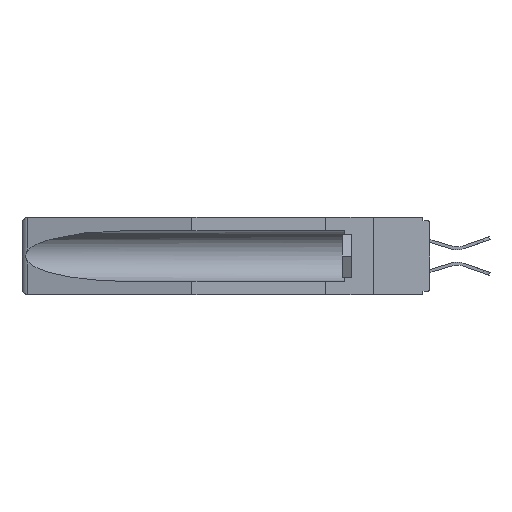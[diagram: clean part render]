
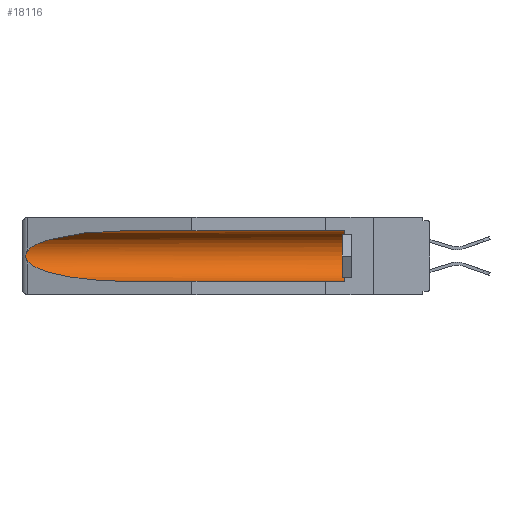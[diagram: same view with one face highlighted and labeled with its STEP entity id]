
A CAD part, left-side view. The second image highlights one B-rep face of the part: STEP entity #18116.
In plain terms, the highlighted cylindrical face has radius 2.857 mm (diameter 5.715 mm), a partial arc.
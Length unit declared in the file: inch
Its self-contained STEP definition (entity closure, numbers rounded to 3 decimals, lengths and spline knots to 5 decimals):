
#35 = CARTESIAN_POINT ( 'NONE',  ( 0.26537, 1.52718, -0.19328 ) ) ;
#506 = CARTESIAN_POINT ( 'NONE',  ( 0.26537, 1.52718, -0.19328 ) ) ;
#765 = CARTESIAN_POINT ( 'NONE',  ( 0.155, 1.07973, -0.059 ) ) ;
#1243 = VERTEX_POINT ( 'NONE', #8244 ) ;
#1831 = VERTEX_POINT ( 'NONE', #11407 ) ;
#2062 = VERTEX_POINT ( 'NONE', #28698 ) ;
#4107 = EDGE_CURVE ( 'NONE', #5020, #1831, #14019, .T. ) ;
#4111 = FACE_OUTER_BOUND ( 'NONE', #20828, .T. ) ;
#4483 = CARTESIAN_POINT ( 'NONE',  ( 0.26537, 1.52718, -0.14972 ) ) ;
#5020 = VERTEX_POINT ( 'NONE', #12432 ) ;
#6721 = CARTESIAN_POINT ( 'NONE',  ( 0.26655, 1.53094, -0.18657 ) ) ;
#6998 = CARTESIAN_POINT ( 'NONE',  ( 0.2675, 1.53308, -0.17534 ) ) ;
#7148 = ORIENTED_EDGE ( 'NONE', *, *, #21753, .T. ) ;
#7287 = CARTESIAN_POINT ( 'NONE',  ( 0.155, -0.30754, -0.284 ) ) ;
#7319 = AXIS2_PLACEMENT_3D ( 'NONE', #10283, #14933, #23999 ) ;
#7691 = VERTEX_POINT ( 'NONE', #10609 ) ;
#8244 = CARTESIAN_POINT ( 'NONE',  ( 0.26537, 1.52718, -0.14972 ) ) ;
#8869 = VERTEX_POINT ( 'NONE', #21587 ) ;
#9433 = EDGE_CURVE ( 'NONE', #1243, #2062, #22752, .T. ) ;
#9462 = EDGE_CURVE ( 'NONE', #2062, #8869, #18335, .T. ) ;
#9974 = CARTESIAN_POINT ( 'NONE',  ( 0.155, -0.30754, -0.059 ) ) ;
#10283 = CARTESIAN_POINT ( 'NONE',  ( 0.155, 0.126, -0.1715 ) ) ;
#10609 = CARTESIAN_POINT ( 'NONE',  ( 0.155, 0.126, -0.284 ) ) ;
#11261 = CARTESIAN_POINT ( 'NONE',  ( 0.26654, 1.53092, -0.15636 ) ) ;
#11364 = CARTESIAN_POINT ( 'NONE',  ( 0.2673, 1.53269, -0.17917 ) ) ;
#11376 = CIRCLE ( 'NONE', #7319, 0.1125 ) ;
#11407 = CARTESIAN_POINT ( 'NONE',  ( 0.155, 1.07973, -0.059 ) ) ;
#11455 = CARTESIAN_POINT ( 'NONE',  ( 0.2673, 1.5327, -0.16383 ) ) ;
#11841 = CARTESIAN_POINT ( 'NONE',  ( 0.155, 1.07973, -0.284 ) ) ;
#12432 = CARTESIAN_POINT ( 'NONE',  ( 0.155, 0.126, -0.059 ) ) ;
#12720 =( BOUNDED_CURVE ( )  B_SPLINE_CURVE ( 3, ( #765, #28111, #14229, #19015 ),
 .UNSPECIFIED., .F., .F. ) 
 B_SPLINE_CURVE_WITH_KNOTS ( ( 4, 4 ),
 ( 4.71239, 6.08839 ),
 .UNSPECIFIED. ) 
 CURVE ( )  GEOMETRIC_REPRESENTATION_ITEM ( )  RATIONAL_B_SPLINE_CURVE ( ( 1., 0.848, 0.848, 1. ) ) 
 REPRESENTATION_ITEM ( '' )  );
#13119 = EDGE_CURVE ( 'NONE', #1831, #1243, #12720, .T. ) ;
#13514 = CARTESIAN_POINT ( 'NONE',  ( 0.2675, 1.53308, -0.16763 ) ) ;
#14019 = LINE ( 'NONE', #9974, #27612 ) ;
#14180 = CARTESIAN_POINT ( 'NONE',  ( 0.21114, 1.30732, -0.284 ) ) ;
#14229 = CARTESIAN_POINT ( 'NONE',  ( 0.25451, 1.48313, -0.09465 ) ) ;
#14885 = DIRECTION ( 'NONE',  ( 0., 0., 1. ) ) ;
#14933 = DIRECTION ( 'NONE',  ( 0., -1., 0. ) ) ;
#15523 = ORIENTED_EDGE ( 'NONE', *, *, #9462, .T. ) ;
#18116 = ADVANCED_FACE ( 'NONE', ( #4111 ), #26829, .F. ) ;
#18335 =( BOUNDED_CURVE ( )  B_SPLINE_CURVE ( 3, ( #506, #22971, #14180, #11841 ),
 .UNSPECIFIED., .F., .F. ) 
 B_SPLINE_CURVE_WITH_KNOTS ( ( 4, 4 ),
 ( 0.1948, 1.5708 ),
 .UNSPECIFIED. ) 
 CURVE ( )  GEOMETRIC_REPRESENTATION_ITEM ( )  RATIONAL_B_SPLINE_CURVE ( ( 1., 0.848, 0.848, 1. ) ) 
 REPRESENTATION_ITEM ( '' )  );
#18692 = DIRECTION ( 'NONE',  ( 0., 1., 0. ) ) ;
#19015 = CARTESIAN_POINT ( 'NONE',  ( 0.26537, 1.52718, -0.14972 ) ) ;
#19338 = CARTESIAN_POINT ( 'NONE',  ( 0.155, -0.30754, -0.1715 ) ) ;
#20357 = ORIENTED_EDGE ( 'NONE', *, *, #9433, .T. ) ;
#20828 = EDGE_LOOP ( 'NONE', ( #27815, #20357, #15523, #23781, #7148, #21472 ) ) ;
#21472 = ORIENTED_EDGE ( 'NONE', *, *, #4107, .T. ) ;
#21587 = CARTESIAN_POINT ( 'NONE',  ( 0.155, 1.07973, -0.284 ) ) ;
#21753 = EDGE_CURVE ( 'NONE', #7691, #5020, #11376, .T. ) ;
#22752 = B_SPLINE_CURVE_WITH_KNOTS ( 'NONE', 3,
 ( #4483, #25091, #11261, #11455, #13514, #6998, #11364, #6721, #24795, #35 ),
 .UNSPECIFIED., .F., .F.,
 ( 4, 2, 2, 2, 4 ),
 ( 0., 0.00029, 0.00058, 0.00087, 0.00117 ),
 .UNSPECIFIED. ) ;
#22971 = CARTESIAN_POINT ( 'NONE',  ( 0.25451, 1.48313, -0.24835 ) ) ;
#23083 = DIRECTION ( 'NONE',  ( 0., 1., 0. ) ) ;
#23647 = DIRECTION ( 'NONE',  ( 0., 1., 0. ) ) ;
#23781 = ORIENTED_EDGE ( 'NONE', *, *, #23882, .F. ) ;
#23811 = AXIS2_PLACEMENT_3D ( 'NONE', #19338, #23647, #14885 ) ;
#23882 = EDGE_CURVE ( 'NONE', #7691, #8869, #24432, .T. ) ;
#23999 = DIRECTION ( 'NONE',  ( 0., 0., 1. ) ) ;
#24432 = LINE ( 'NONE', #7287, #25841 ) ;
#24795 = CARTESIAN_POINT ( 'NONE',  ( 0.26597, 1.5296, -0.19026 ) ) ;
#25091 = CARTESIAN_POINT ( 'NONE',  ( 0.26597, 1.52961, -0.15275 ) ) ;
#25841 = VECTOR ( 'NONE', #23083, 39.37008 ) ;
#26829 = CYLINDRICAL_SURFACE ( 'NONE', #23811, 0.1125 ) ;
#27612 = VECTOR ( 'NONE', #18692, 39.37008 ) ;
#27815 = ORIENTED_EDGE ( 'NONE', *, *, #13119, .T. ) ;
#28111 = CARTESIAN_POINT ( 'NONE',  ( 0.21114, 1.30732, -0.059 ) ) ;
#28698 = CARTESIAN_POINT ( 'NONE',  ( 0.26537, 1.52718, -0.19328 ) ) ;
